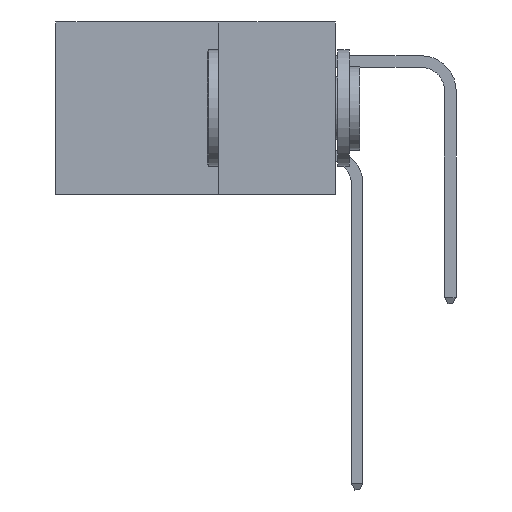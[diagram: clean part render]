
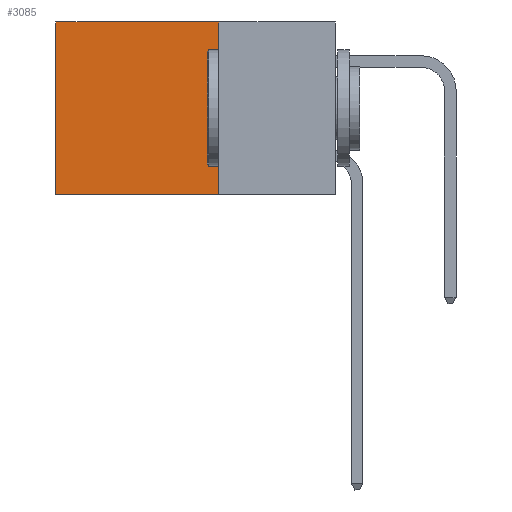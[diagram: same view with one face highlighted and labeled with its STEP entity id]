
A CAD part, left-side view. The second image highlights one B-rep face of the part: STEP entity #3085.
In plain terms, the highlighted planar face has unit normal (-1, 0, 0).
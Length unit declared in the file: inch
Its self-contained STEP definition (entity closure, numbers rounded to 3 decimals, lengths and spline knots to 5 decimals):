
#42 = CARTESIAN_POINT ( 'NONE',  ( 0.2875, 0.25, 0. ) ) ;
#560 = CARTESIAN_POINT ( 'NONE',  ( 0.2875, 0.6, 0. ) ) ;
#665 = VERTEX_POINT ( 'NONE', #11396 ) ;
#1704 = ORIENTED_EDGE ( 'NONE', *, *, #2528, .T. ) ;
#2528 = EDGE_CURVE ( 'NONE', #5234, #8798, #5915, .T. ) ;
#3085 = ADVANCED_FACE ( 'NONE', ( #15316 ), #16892, .F. ) ;
#3173 = ORIENTED_EDGE ( 'NONE', *, *, #4132, .F. ) ;
#4046 = CARTESIAN_POINT ( 'NONE',  ( 0.2875, 0.25, 0. ) ) ;
#4132 = EDGE_CURVE ( 'NONE', #665, #8798, #13127, .T. ) ;
#4950 = AXIS2_PLACEMENT_3D ( 'NONE', #8669, #10307, #6018 ) ;
#5214 = VECTOR ( 'NONE', #12902, 39.37008 ) ;
#5234 = VERTEX_POINT ( 'NONE', #6874 ) ;
#5915 = LINE ( 'NONE', #560, #8660 ) ;
#6018 = DIRECTION ( 'NONE',  ( 0., 0., -1. ) ) ;
#6874 = CARTESIAN_POINT ( 'NONE',  ( 0.2875, 0.6, 0. ) ) ;
#8660 = VECTOR ( 'NONE', #14262, 39.37008 ) ;
#8669 = CARTESIAN_POINT ( 'NONE',  ( 0.2875, 0.25, 0. ) ) ;
#8798 = VERTEX_POINT ( 'NONE', #16569 ) ;
#10307 = DIRECTION ( 'NONE',  ( 1., 0., 0. ) ) ;
#10323 = ORIENTED_EDGE ( 'NONE', *, *, #15442, .T. ) ;
#10652 = VECTOR ( 'NONE', #15042, 39.37008 ) ;
#10939 = EDGE_LOOP ( 'NONE', ( #1704, #3173, #10989, #10323 ) ) ;
#10989 = ORIENTED_EDGE ( 'NONE', *, *, #12318, .F. ) ;
#11396 = CARTESIAN_POINT ( 'NONE',  ( 0.2875, 0.25, -0.37 ) ) ;
#11627 = CARTESIAN_POINT ( 'NONE',  ( 0.2875, 0.25, -0.37 ) ) ;
#12318 = EDGE_CURVE ( 'NONE', #15850, #665, #15598, .T. ) ;
#12325 = DIRECTION ( 'NONE',  ( 0., 0., -1. ) ) ;
#12902 = DIRECTION ( 'NONE',  ( 0., 1., 0. ) ) ;
#13127 = LINE ( 'NONE', #11627, #5214 ) ;
#14262 = DIRECTION ( 'NONE',  ( 0., 0., -1. ) ) ;
#14933 = LINE ( 'NONE', #4046, #10652 ) ;
#15042 = DIRECTION ( 'NONE',  ( 0., 1., 0. ) ) ;
#15316 = FACE_OUTER_BOUND ( 'NONE', #10939, .T. ) ;
#15442 = EDGE_CURVE ( 'NONE', #15850, #5234, #14933, .T. ) ;
#15598 = LINE ( 'NONE', #42, #16049 ) ;
#15850 = VERTEX_POINT ( 'NONE', #17296 ) ;
#16049 = VECTOR ( 'NONE', #12325, 39.37008 ) ;
#16569 = CARTESIAN_POINT ( 'NONE',  ( 0.2875, 0.6, -0.37 ) ) ;
#16892 = PLANE ( 'NONE',  #4950 ) ;
#17296 = CARTESIAN_POINT ( 'NONE',  ( 0.2875, 0.25, 0. ) ) ;
